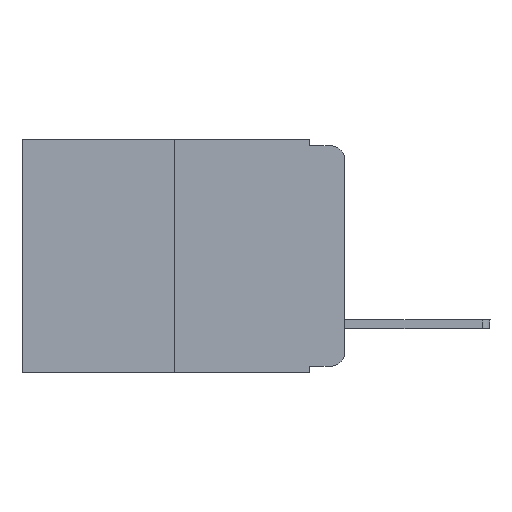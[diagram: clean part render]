
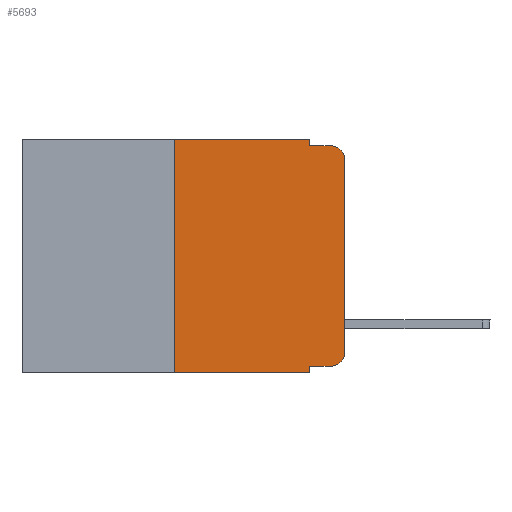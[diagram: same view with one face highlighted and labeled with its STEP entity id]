
A CAD part, left-side view. The second image highlights one B-rep face of the part: STEP entity #5693.
In plain terms, the highlighted planar face has unit normal (-1, 0, 0).
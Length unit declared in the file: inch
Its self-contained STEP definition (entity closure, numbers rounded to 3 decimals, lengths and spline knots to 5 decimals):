
#49 = CARTESIAN_POINT ( 'NONE',  ( 0., 0., -0.313 ) ) ;
#77 = DIRECTION ( 'NONE',  ( 0., 0., -1. ) ) ;
#1077 = DIRECTION ( 'NONE',  ( 0., 0., 1. ) ) ;
#1342 = VECTOR ( 'NONE', #2727, 39.37008 ) ;
#1751 = VERTEX_POINT ( 'NONE', #15332 ) ;
#1995 = DIRECTION ( 'NONE',  ( 1., 0., 0. ) ) ;
#2485 = VERTEX_POINT ( 'NONE', #8016 ) ;
#2727 = DIRECTION ( 'NONE',  ( 0., -1., 0. ) ) ;
#3221 = VERTEX_POINT ( 'NONE', #15506 ) ;
#3896 = CARTESIAN_POINT ( 'NONE',  ( 0., 0.02, -0.333 ) ) ;
#4587 = AXIS2_PLACEMENT_3D ( 'NONE', #5224, #16587, #20241 ) ;
#4649 = LINE ( 'NONE', #22316, #22682 ) ;
#4994 = ORIENTED_EDGE ( 'NONE', *, *, #20365, .T. ) ;
#5224 = CARTESIAN_POINT ( 'NONE',  ( 0., 0.02, -0.313 ) ) ;
#5421 = EDGE_CURVE ( 'NONE', #24234, #1751, #4649, .T. ) ;
#5662 = EDGE_CURVE ( 'NONE', #12945, #15368, #13608, .T. ) ;
#5693 = ADVANCED_FACE ( 'NONE', ( #13725 ), #9805, .F. ) ;
#5813 = CIRCLE ( 'NONE', #4587, 0.02 ) ;
#5855 = EDGE_CURVE ( 'NONE', #12945, #14586, #14209, .T. ) ;
#5912 = EDGE_CURVE ( 'NONE', #1751, #2485, #12691, .T. ) ;
#6351 = DIRECTION ( 'NONE',  ( 0., 0., -1. ) ) ;
#6912 = VECTOR ( 'NONE', #15868, 39.37008 ) ;
#7014 = ORIENTED_EDGE ( 'NONE', *, *, #5662, .T. ) ;
#7408 = VECTOR ( 'NONE', #6351, 39.37008 ) ;
#8010 = CARTESIAN_POINT ( 'NONE',  ( 0., 0.051, 0. ) ) ;
#8016 = CARTESIAN_POINT ( 'NONE',  ( 0., 0.051, 0. ) ) ;
#8145 = AXIS2_PLACEMENT_3D ( 'NONE', #17757, #1995, #77 ) ;
#8657 = ORIENTED_EDGE ( 'NONE', *, *, #5912, .F. ) ;
#9084 = LINE ( 'NONE', #18928, #24310 ) ;
#9347 = ORIENTED_EDGE ( 'NONE', *, *, #5421, .F. ) ;
#9502 = DIRECTION ( 'NONE',  ( 0., 0., -1. ) ) ;
#9708 = DIRECTION ( 'NONE',  ( 0., -1., 0. ) ) ;
#9740 = EDGE_CURVE ( 'NONE', #16861, #3221, #14646, .T. ) ;
#9805 = PLANE ( 'NONE',  #8145 ) ;
#9935 = CARTESIAN_POINT ( 'NONE',  ( 0., 0.051, -0.333 ) ) ;
#10712 = EDGE_LOOP ( 'NONE', ( #20336, #13740, #21388, #18044, #8657, #9347, #19031, #15676, #7014, #4994 ) ) ;
#11805 = LINE ( 'NONE', #8010, #7408 ) ;
#12116 = VECTOR ( 'NONE', #1077, 39.37008 ) ;
#12438 = CARTESIAN_POINT ( 'NONE',  ( 0., 0.051, 0. ) ) ;
#12691 = LINE ( 'NONE', #16235, #1342 ) ;
#12945 = VERTEX_POINT ( 'NONE', #22174 ) ;
#13399 = CARTESIAN_POINT ( 'NONE',  ( 0., 0.02, -0.03 ) ) ;
#13608 = LINE ( 'NONE', #9935, #6912 ) ;
#13725 = FACE_OUTER_BOUND ( 'NONE', #10712, .T. ) ;
#13740 = ORIENTED_EDGE ( 'NONE', *, *, #9740, .T. ) ;
#13767 = EDGE_CURVE ( 'NONE', #20651, #3221, #16542, .T. ) ;
#13781 = DIRECTION ( 'NONE',  ( -1., 0., 0. ) ) ;
#14209 = LINE ( 'NONE', #12438, #17481 ) ;
#14582 = CARTESIAN_POINT ( 'NONE',  ( 0., 0.051, -0.343 ) ) ;
#14586 = VERTEX_POINT ( 'NONE', #14582 ) ;
#14646 = CIRCLE ( 'NONE', #15106, 0.02 ) ;
#15106 = AXIS2_PLACEMENT_3D ( 'NONE', #13399, #13781, #9502 ) ;
#15332 = CARTESIAN_POINT ( 'NONE',  ( 0., 0.25, 0. ) ) ;
#15368 = VERTEX_POINT ( 'NONE', #3896 ) ;
#15506 = CARTESIAN_POINT ( 'NONE',  ( 0., 0.02, -0.01 ) ) ;
#15630 = EDGE_CURVE ( 'NONE', #23813, #16861, #18380, .T. ) ;
#15676 = ORIENTED_EDGE ( 'NONE', *, *, #5855, .F. ) ;
#15868 = DIRECTION ( 'NONE',  ( 0., -1., 0. ) ) ;
#16235 = CARTESIAN_POINT ( 'NONE',  ( 0., 0.473, 0. ) ) ;
#16482 = DIRECTION ( 'NONE',  ( 0., 0., -1. ) ) ;
#16542 = LINE ( 'NONE', #17047, #20933 ) ;
#16587 = DIRECTION ( 'NONE',  ( -1., 0., 0. ) ) ;
#16861 = VERTEX_POINT ( 'NONE', #20026 ) ;
#17047 = CARTESIAN_POINT ( 'NONE',  ( 0., 0.051, -0.01 ) ) ;
#17326 = CARTESIAN_POINT ( 'NONE',  ( 0., 0., 0. ) ) ;
#17481 = VECTOR ( 'NONE', #16482, 39.37008 ) ;
#17757 = CARTESIAN_POINT ( 'NONE',  ( 0., 0.473, 0. ) ) ;
#17887 = EDGE_CURVE ( 'NONE', #24234, #14586, #9084, .T. ) ;
#18044 = ORIENTED_EDGE ( 'NONE', *, *, #20227, .F. ) ;
#18380 = LINE ( 'NONE', #17326, #12116 ) ;
#18928 = CARTESIAN_POINT ( 'NONE',  ( 0., 0.473, -0.343 ) ) ;
#19031 = ORIENTED_EDGE ( 'NONE', *, *, #17887, .T. ) ;
#19103 = CARTESIAN_POINT ( 'NONE',  ( 0., 0.25, -0.343 ) ) ;
#19613 = CARTESIAN_POINT ( 'NONE',  ( 0., 0.051, -0.01 ) ) ;
#20026 = CARTESIAN_POINT ( 'NONE',  ( 0., 0., -0.03 ) ) ;
#20227 = EDGE_CURVE ( 'NONE', #2485, #20651, #11805, .T. ) ;
#20241 = DIRECTION ( 'NONE',  ( 0., 0., -1. ) ) ;
#20336 = ORIENTED_EDGE ( 'NONE', *, *, #15630, .T. ) ;
#20365 = EDGE_CURVE ( 'NONE', #15368, #23813, #5813, .T. ) ;
#20651 = VERTEX_POINT ( 'NONE', #19613 ) ;
#20933 = VECTOR ( 'NONE', #9708, 39.37008 ) ;
#21388 = ORIENTED_EDGE ( 'NONE', *, *, #13767, .F. ) ;
#22056 = DIRECTION ( 'NONE',  ( 0., 0., 1. ) ) ;
#22174 = CARTESIAN_POINT ( 'NONE',  ( 0., 0.051, -0.333 ) ) ;
#22316 = CARTESIAN_POINT ( 'NONE',  ( 0., 0.25, 0. ) ) ;
#22584 = DIRECTION ( 'NONE',  ( 0., -1., 0. ) ) ;
#22682 = VECTOR ( 'NONE', #22056, 39.37008 ) ;
#23813 = VERTEX_POINT ( 'NONE', #49 ) ;
#24234 = VERTEX_POINT ( 'NONE', #19103 ) ;
#24310 = VECTOR ( 'NONE', #22584, 39.37008 ) ;
